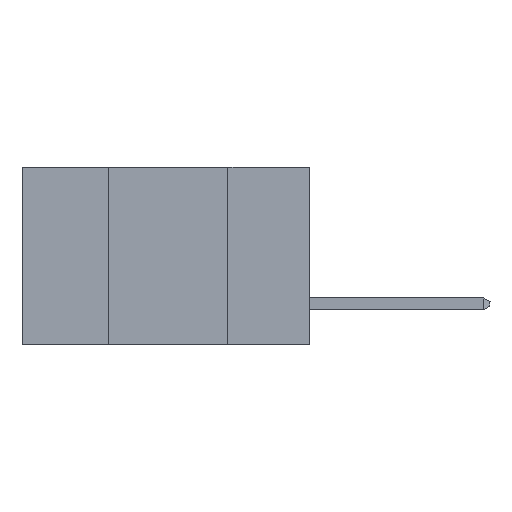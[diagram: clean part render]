
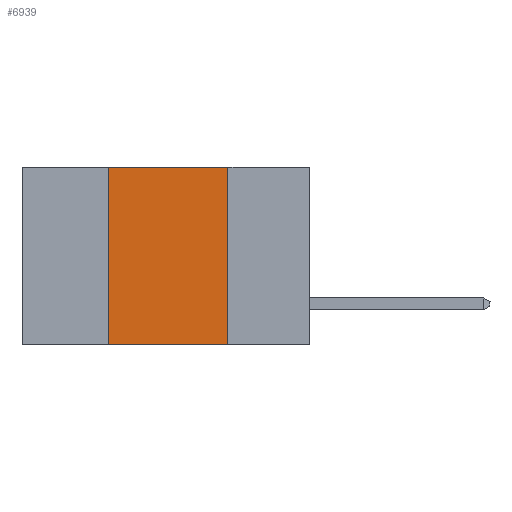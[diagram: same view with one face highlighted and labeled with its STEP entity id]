
A CAD part, left-side view. The second image highlights one B-rep face of the part: STEP entity #6939.
In plain terms, the highlighted planar face has unit normal (-1, 0, 0).
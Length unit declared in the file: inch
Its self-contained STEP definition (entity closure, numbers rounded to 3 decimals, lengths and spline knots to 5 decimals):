
#293 = DIRECTION ( 'NONE',  ( 0., -1., 0. ) ) ;
#596 = DIRECTION ( 'NONE',  ( 0., 0., -1. ) ) ;
#4161 = DIRECTION ( 'NONE',  ( 0., 0., -1. ) ) ;
#5894 = LINE ( 'NONE', #44756, #18552 ) ;
#6255 = LINE ( 'NONE', #11555, #43422 ) ;
#6939 = ADVANCED_FACE ( 'NONE', ( #48857 ), #34652, .F. ) ;
#7159 = LINE ( 'NONE', #23865, #24531 ) ;
#9831 = CARTESIAN_POINT ( 'NONE',  ( 0., 0.6, -0.37 ) ) ;
#10244 = ORIENTED_EDGE ( 'NONE', *, *, #43009, .T. ) ;
#11555 = CARTESIAN_POINT ( 'NONE',  ( 0., 0.6, 0. ) ) ;
#13601 = EDGE_CURVE ( 'NONE', #38037, #47680, #5894, .T. ) ;
#14094 = ORIENTED_EDGE ( 'NONE', *, *, #22000, .F. ) ;
#14140 = VERTEX_POINT ( 'NONE', #27648 ) ;
#17677 = EDGE_CURVE ( 'NONE', #14140, #20420, #7159, .T. ) ;
#18552 = VECTOR ( 'NONE', #48259, 39.37008 ) ;
#20420 = VERTEX_POINT ( 'NONE', #39606 ) ;
#22000 = EDGE_CURVE ( 'NONE', #47680, #14140, #6255, .T. ) ;
#22231 = EDGE_LOOP ( 'NONE', ( #48658, #14094, #33991, #10244 ) ) ;
#22278 = CARTESIAN_POINT ( 'NONE',  ( 0., 0.42, 0. ) ) ;
#23865 = CARTESIAN_POINT ( 'NONE',  ( 0., 0.17, 0. ) ) ;
#24531 = VECTOR ( 'NONE', #596, 39.37008 ) ;
#25056 = DIRECTION ( 'NONE',  ( 0., -1., 0. ) ) ;
#27104 = DIRECTION ( 'NONE',  ( 1., 0., 0. ) ) ;
#27648 = CARTESIAN_POINT ( 'NONE',  ( 0., 0.17, 0. ) ) ;
#29722 = VECTOR ( 'NONE', #25056, 39.37008 ) ;
#33332 = LINE ( 'NONE', #9831, #29722 ) ;
#33991 = ORIENTED_EDGE ( 'NONE', *, *, #13601, .F. ) ;
#34652 = PLANE ( 'NONE',  #34730 ) ;
#34730 = AXIS2_PLACEMENT_3D ( 'NONE', #46182, #27104, #4161 ) ;
#38037 = VERTEX_POINT ( 'NONE', #43937 ) ;
#39606 = CARTESIAN_POINT ( 'NONE',  ( 0., 0.17, -0.37 ) ) ;
#43009 = EDGE_CURVE ( 'NONE', #38037, #20420, #33332, .T. ) ;
#43422 = VECTOR ( 'NONE', #293, 39.37008 ) ;
#43937 = CARTESIAN_POINT ( 'NONE',  ( 0., 0.42, -0.37 ) ) ;
#44756 = CARTESIAN_POINT ( 'NONE',  ( 0., 0.42, 0. ) ) ;
#46182 = CARTESIAN_POINT ( 'NONE',  ( 0., 0.6, 0. ) ) ;
#47680 = VERTEX_POINT ( 'NONE', #22278 ) ;
#48259 = DIRECTION ( 'NONE',  ( 0., 0., 1. ) ) ;
#48658 = ORIENTED_EDGE ( 'NONE', *, *, #17677, .F. ) ;
#48857 = FACE_OUTER_BOUND ( 'NONE', #22231, .T. ) ;
